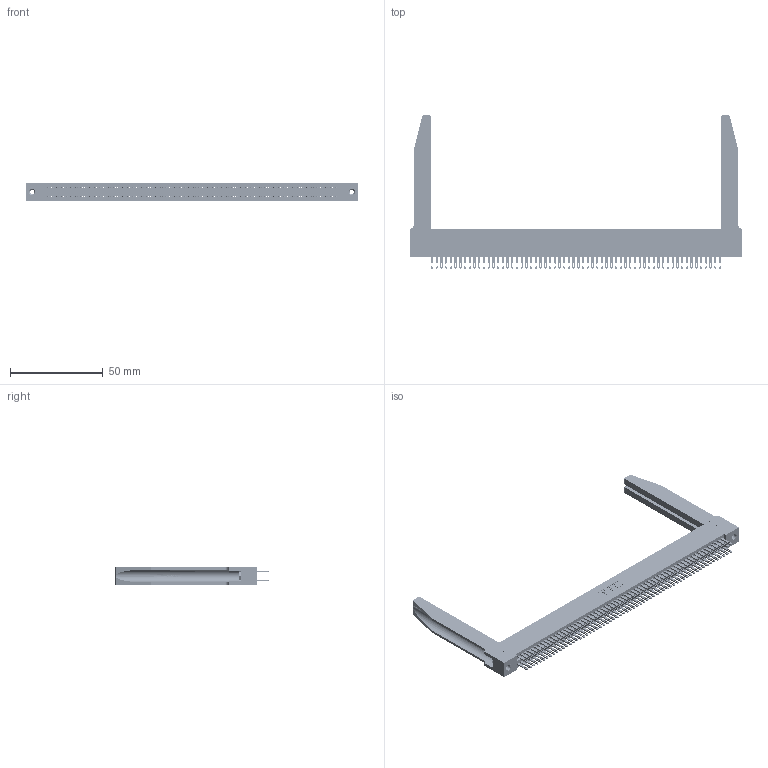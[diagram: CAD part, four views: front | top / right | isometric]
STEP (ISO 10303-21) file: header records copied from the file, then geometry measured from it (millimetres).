
FILE_DESCRIPTION (( 'STEP AP203' ), '1' );
FILE_NAME ('345-124-500-278.STEP', '2019-11-06T16:36:57', ( '' ), ( '' ), 'SwSTEP 2.0', 'SolidWorks 2016', '' );
FILE_SCHEMA (( 'CONFIG_CONTROL_DESIGN' ));
Length unit declared in the file: inch
Products named in the file (5): 345-124-500-278; 345-250-001_345-250-001-102; 345-220-078_345-220-078; 345-292-001_345-293-100; 345 Part_Flush Mounting Lugs - 0.156 Dia-TH
Assembly tree (129 placements, depth 2):
  345-124-500-278
    345 Part_Flush Mounting Lugs - 0.156 Dia-TH
    345-292-001_345-293-100  x124
    345-250-001_345-250-001-102  x2
    345-220-078_345-220-078  x2
Bounding box: 178.71 x 82.47 x 9.4 mm (x, y, z)
Volume: 25695.5 mm3; surface area: 34986.8 mm2
Topology: 129 solids, 129 shells, 6064 faces, 18433 edges, 12278 vertices
Faces by surface type: plane 3570, cylinder 2442, bspline 36, cone 12, torus 4
Entity records: 50624 total; most frequent: CARTESIAN_POINT 9383, ORIENTED_EDGE 8214, DIRECTION 7245, EDGE_CURVE 4107, VECTOR 3629, LINE 3629, VERTEX_POINT 2732, AXIS2_PLACEMENT_3D 1808
